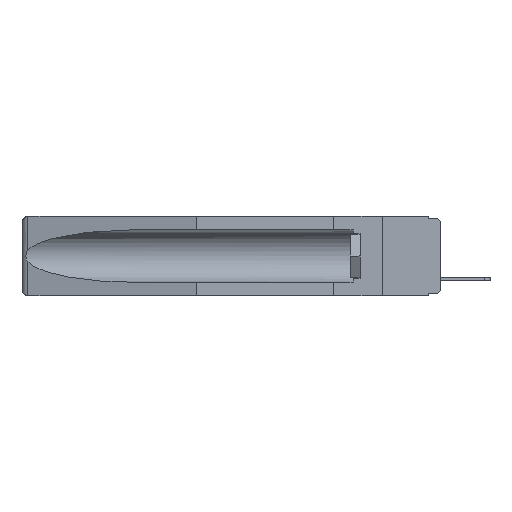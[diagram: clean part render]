
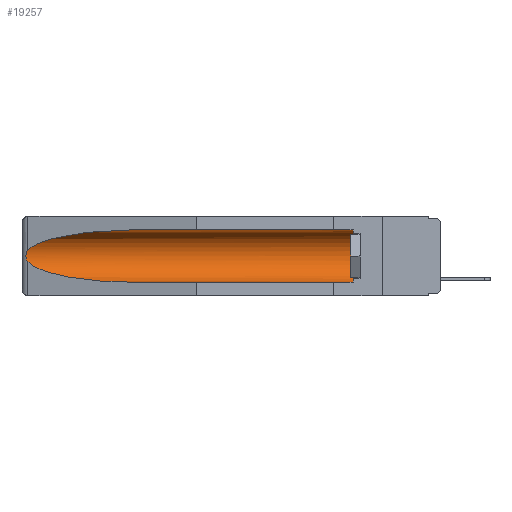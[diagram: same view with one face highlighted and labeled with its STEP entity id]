
A CAD part, left-side view. The second image highlights one B-rep face of the part: STEP entity #19257.
In plain terms, the highlighted cylindrical face has radius 2.857 mm (diameter 5.715 mm), a partial arc.
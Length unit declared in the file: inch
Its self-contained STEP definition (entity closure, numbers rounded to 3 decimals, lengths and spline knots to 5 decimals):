
#47 = EDGE_CURVE ( 'NONE', #7250, #13510, #6664, .T. ) ;
#230 = VECTOR ( 'NONE', #5575, 39.37008 ) ;
#304 = CARTESIAN_POINT ( 'NONE',  ( 0.155, 1.07973, -0.284 ) ) ;
#613 = CARTESIAN_POINT ( 'NONE',  ( 0.155, 0.126, -0.284 ) ) ;
#713 = CARTESIAN_POINT ( 'NONE',  ( 0.26537, 1.52718, -0.14972 ) ) ;
#907 = DIRECTION ( 'NONE',  ( 0., -1., 0. ) ) ;
#973 = LINE ( 'NONE', #5568, #10823 ) ;
#1110 = CARTESIAN_POINT ( 'NONE',  ( 0.26537, 1.52718, -0.19328 ) ) ;
#1239 = VERTEX_POINT ( 'NONE', #613 ) ;
#3926 = DIRECTION ( 'NONE',  ( 0., 0., 1. ) ) ;
#4163 = CARTESIAN_POINT ( 'NONE',  ( 0.26537, 1.52718, -0.14972 ) ) ;
#4182 = CARTESIAN_POINT ( 'NONE',  ( 0.26537, 1.52718, -0.19328 ) ) ;
#4402 = CARTESIAN_POINT ( 'NONE',  ( 0.155, -0.30754, -0.059 ) ) ;
#4525 = ORIENTED_EDGE ( 'NONE', *, *, #13971, .T. ) ;
#4678 = LINE ( 'NONE', #4402, #230 ) ;
#5443 = AXIS2_PLACEMENT_3D ( 'NONE', #17339, #9887, #3926 ) ;
#5568 = CARTESIAN_POINT ( 'NONE',  ( 0.155, -0.30754, -0.284 ) ) ;
#5575 = DIRECTION ( 'NONE',  ( 0., 1., 0. ) ) ;
#5703 = CARTESIAN_POINT ( 'NONE',  ( 0.21114, 1.30732, -0.059 ) ) ;
#5813 = B_SPLINE_CURVE_WITH_KNOTS ( 'NONE', 3,
 ( #4163, #14606, #17518, #14725, #8610, #7196, #11589, #7257, #7131, #1110 ),
 .UNSPECIFIED., .F., .F.,
 ( 4, 2, 2, 2, 4 ),
 ( 0., 0.00029, 0.00058, 0.00087, 0.00117 ),
 .UNSPECIFIED. ) ;
#5958 = CARTESIAN_POINT ( 'NONE',  ( 0.25451, 1.48313, -0.09465 ) ) ;
#6664 =( BOUNDED_CURVE ( )  B_SPLINE_CURVE ( 3, ( #15581, #9610, #15766, #17249 ),
 .UNSPECIFIED., .F., .F. ) 
 B_SPLINE_CURVE_WITH_KNOTS ( ( 4, 4 ),
 ( 0.1948, 1.5708 ),
 .UNSPECIFIED. ) 
 CURVE ( )  GEOMETRIC_REPRESENTATION_ITEM ( )  RATIONAL_B_SPLINE_CURVE ( ( 1., 0.848, 0.848, 1. ) ) 
 REPRESENTATION_ITEM ( '' )  );
#7131 = CARTESIAN_POINT ( 'NONE',  ( 0.26597, 1.5296, -0.19026 ) ) ;
#7196 = CARTESIAN_POINT ( 'NONE',  ( 0.2675, 1.53308, -0.17534 ) ) ;
#7250 = VERTEX_POINT ( 'NONE', #4182 ) ;
#7257 = CARTESIAN_POINT ( 'NONE',  ( 0.26655, 1.53094, -0.18657 ) ) ;
#8610 = CARTESIAN_POINT ( 'NONE',  ( 0.2675, 1.53308, -0.16763 ) ) ;
#8733 = CARTESIAN_POINT ( 'NONE',  ( 0.155, 1.07973, -0.059 ) ) ;
#9610 = CARTESIAN_POINT ( 'NONE',  ( 0.25451, 1.48313, -0.24835 ) ) ;
#9887 = DIRECTION ( 'NONE',  ( 0., 1., 0. ) ) ;
#10545 = CARTESIAN_POINT ( 'NONE',  ( 0.26537, 1.52718, -0.14972 ) ) ;
#10593 = ORIENTED_EDGE ( 'NONE', *, *, #14844, .T. ) ;
#10823 = VECTOR ( 'NONE', #18908, 39.37008 ) ;
#11193 = EDGE_CURVE ( 'NONE', #1239, #13510, #973, .T. ) ;
#11495 = ORIENTED_EDGE ( 'NONE', *, *, #11193, .F. ) ;
#11589 = CARTESIAN_POINT ( 'NONE',  ( 0.2673, 1.53269, -0.17917 ) ) ;
#12329 = VERTEX_POINT ( 'NONE', #8733 ) ;
#12820 = CIRCLE ( 'NONE', #13453, 0.1125 ) ;
#13260 = ORIENTED_EDGE ( 'NONE', *, *, #47, .T. ) ;
#13453 = AXIS2_PLACEMENT_3D ( 'NONE', #15829, #907, #18680 ) ;
#13510 = VERTEX_POINT ( 'NONE', #304 ) ;
#13971 = EDGE_CURVE ( 'NONE', #19278, #12329, #4678, .T. ) ;
#14280 = FACE_OUTER_BOUND ( 'NONE', #16565, .T. ) ;
#14606 = CARTESIAN_POINT ( 'NONE',  ( 0.26597, 1.52961, -0.15275 ) ) ;
#14725 = CARTESIAN_POINT ( 'NONE',  ( 0.2673, 1.5327, -0.16383 ) ) ;
#14844 = EDGE_CURVE ( 'NONE', #12329, #15149, #18521, .T. ) ;
#15149 = VERTEX_POINT ( 'NONE', #713 ) ;
#15253 = EDGE_CURVE ( 'NONE', #1239, #19278, #12820, .T. ) ;
#15362 = EDGE_CURVE ( 'NONE', #15149, #7250, #5813, .T. ) ;
#15581 = CARTESIAN_POINT ( 'NONE',  ( 0.26537, 1.52718, -0.19328 ) ) ;
#15678 = CYLINDRICAL_SURFACE ( 'NONE', #5443, 0.1125 ) ;
#15766 = CARTESIAN_POINT ( 'NONE',  ( 0.21114, 1.30732, -0.284 ) ) ;
#15829 = CARTESIAN_POINT ( 'NONE',  ( 0.155, 0.126, -0.1715 ) ) ;
#16565 = EDGE_LOOP ( 'NONE', ( #10593, #17489, #13260, #11495, #17030, #4525 ) ) ;
#17030 = ORIENTED_EDGE ( 'NONE', *, *, #15253, .T. ) ;
#17249 = CARTESIAN_POINT ( 'NONE',  ( 0.155, 1.07973, -0.284 ) ) ;
#17339 = CARTESIAN_POINT ( 'NONE',  ( 0.155, -0.30754, -0.1715 ) ) ;
#17473 = CARTESIAN_POINT ( 'NONE',  ( 0.155, 0.126, -0.059 ) ) ;
#17489 = ORIENTED_EDGE ( 'NONE', *, *, #15362, .T. ) ;
#17518 = CARTESIAN_POINT ( 'NONE',  ( 0.26654, 1.53092, -0.15636 ) ) ;
#17606 = CARTESIAN_POINT ( 'NONE',  ( 0.155, 1.07973, -0.059 ) ) ;
#18521 =( BOUNDED_CURVE ( )  B_SPLINE_CURVE ( 3, ( #17606, #5703, #5958, #10545 ),
 .UNSPECIFIED., .F., .F. ) 
 B_SPLINE_CURVE_WITH_KNOTS ( ( 4, 4 ),
 ( 4.71239, 6.08839 ),
 .UNSPECIFIED. ) 
 CURVE ( )  GEOMETRIC_REPRESENTATION_ITEM ( )  RATIONAL_B_SPLINE_CURVE ( ( 1., 0.848, 0.848, 1. ) ) 
 REPRESENTATION_ITEM ( '' )  );
#18680 = DIRECTION ( 'NONE',  ( 0., 0., 1. ) ) ;
#18908 = DIRECTION ( 'NONE',  ( 0., 1., 0. ) ) ;
#19257 = ADVANCED_FACE ( 'NONE', ( #14280 ), #15678, .F. ) ;
#19278 = VERTEX_POINT ( 'NONE', #17473 ) ;
